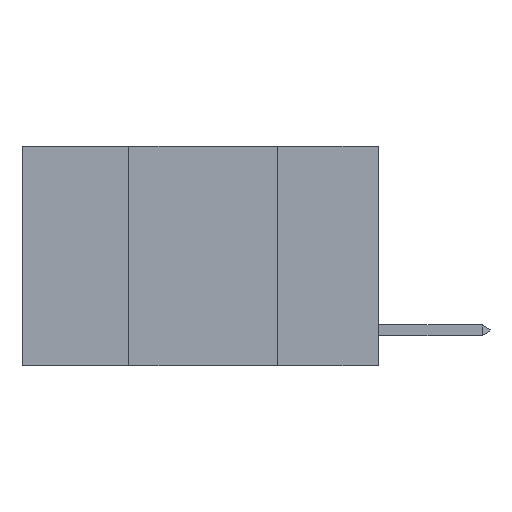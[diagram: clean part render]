
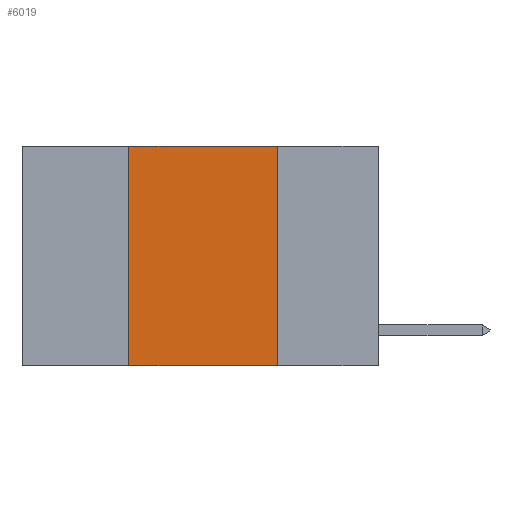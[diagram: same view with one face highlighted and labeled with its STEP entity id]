
A CAD part, left-side view. The second image highlights one B-rep face of the part: STEP entity #6019.
In plain terms, the highlighted planar face has unit normal (-1, 0, 0).
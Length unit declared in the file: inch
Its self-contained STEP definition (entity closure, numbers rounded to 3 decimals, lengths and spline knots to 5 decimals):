
#269 = CARTESIAN_POINT ( 'NONE',  ( 0., 0.6, 0. ) ) ;
#1616 = DIRECTION ( 'NONE',  ( 0., -1., 0. ) ) ;
#1897 = VECTOR ( 'NONE', #2283, 39.37008 ) ;
#2035 = DIRECTION ( 'NONE',  ( 0., 0., -1. ) ) ;
#2283 = DIRECTION ( 'NONE',  ( 0., -1., 0. ) ) ;
#2758 = ORIENTED_EDGE ( 'NONE', *, *, #11259, .F. ) ;
#3228 = LINE ( 'NONE', #17425, #6484 ) ;
#3525 = VERTEX_POINT ( 'NONE', #11846 ) ;
#3816 = LINE ( 'NONE', #12113, #12692 ) ;
#3960 = CARTESIAN_POINT ( 'NONE',  ( 0., 0.42, -0.37 ) ) ;
#4332 = CARTESIAN_POINT ( 'NONE',  ( 0., 0.6, -0.37 ) ) ;
#4752 = EDGE_CURVE ( 'NONE', #3525, #8467, #3228, .T. ) ;
#6019 = ADVANCED_FACE ( 'NONE', ( #18739 ), #24830, .F. ) ;
#6125 = AXIS2_PLACEMENT_3D ( 'NONE', #269, #22388, #22665 ) ;
#6484 = VECTOR ( 'NONE', #1616, 39.37008 ) ;
#7179 = DIRECTION ( 'NONE',  ( 0., 0., 1. ) ) ;
#7250 = ORIENTED_EDGE ( 'NONE', *, *, #24124, .T. ) ;
#8467 = VERTEX_POINT ( 'NONE', #15880 ) ;
#11259 = EDGE_CURVE ( 'NONE', #18937, #3525, #16536, .T. ) ;
#11846 = CARTESIAN_POINT ( 'NONE',  ( 0., 0.42, 0. ) ) ;
#12113 = CARTESIAN_POINT ( 'NONE',  ( 0., 0.17, 0. ) ) ;
#12692 = VECTOR ( 'NONE', #2035, 39.37008 ) ;
#14959 = EDGE_LOOP ( 'NONE', ( #16467, #25830, #2758, #7250 ) ) ;
#15456 = CARTESIAN_POINT ( 'NONE',  ( 0., 0.42, 0. ) ) ;
#15880 = CARTESIAN_POINT ( 'NONE',  ( 0., 0.17, 0. ) ) ;
#16467 = ORIENTED_EDGE ( 'NONE', *, *, #25398, .F. ) ;
#16505 = CARTESIAN_POINT ( 'NONE',  ( 0., 0.17, -0.37 ) ) ;
#16536 = LINE ( 'NONE', #15456, #17034 ) ;
#17034 = VECTOR ( 'NONE', #7179, 39.37008 ) ;
#17425 = CARTESIAN_POINT ( 'NONE',  ( 0., 0.6, 0. ) ) ;
#17861 = LINE ( 'NONE', #4332, #1897 ) ;
#18739 = FACE_OUTER_BOUND ( 'NONE', #14959, .T. ) ;
#18937 = VERTEX_POINT ( 'NONE', #3960 ) ;
#22388 = DIRECTION ( 'NONE',  ( 1., 0., 0. ) ) ;
#22665 = DIRECTION ( 'NONE',  ( 0., 0., -1. ) ) ;
#23010 = VERTEX_POINT ( 'NONE', #16505 ) ;
#24124 = EDGE_CURVE ( 'NONE', #18937, #23010, #17861, .T. ) ;
#24830 = PLANE ( 'NONE',  #6125 ) ;
#25398 = EDGE_CURVE ( 'NONE', #8467, #23010, #3816, .T. ) ;
#25830 = ORIENTED_EDGE ( 'NONE', *, *, #4752, .F. ) ;
